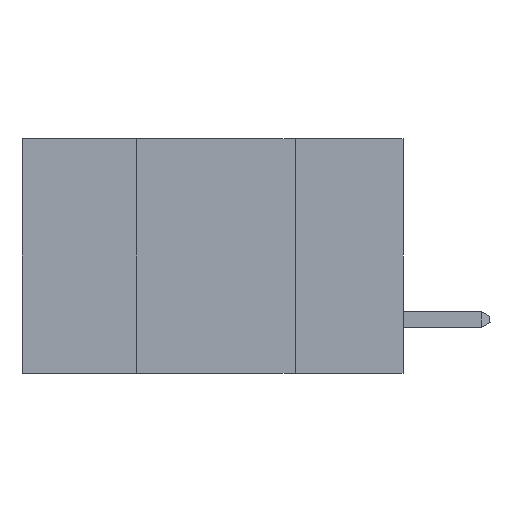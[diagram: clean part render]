
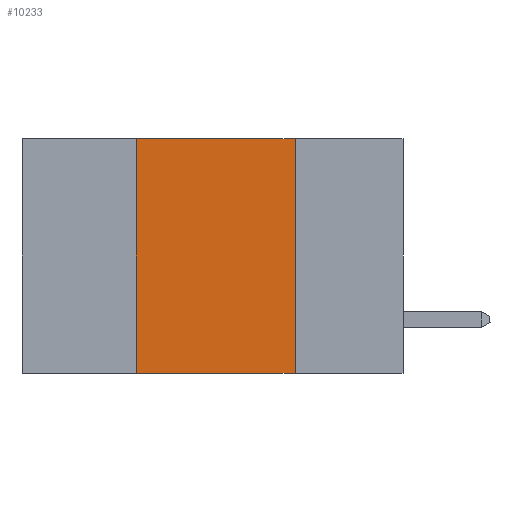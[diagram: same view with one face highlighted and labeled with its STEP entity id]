
A CAD part, left-side view. The second image highlights one B-rep face of the part: STEP entity #10233.
In plain terms, the highlighted planar face has unit normal (-1, 0, 0).
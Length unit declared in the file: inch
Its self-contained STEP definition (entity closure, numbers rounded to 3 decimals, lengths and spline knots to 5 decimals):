
#122 = CARTESIAN_POINT ( 'NONE',  ( 0., 0.42, 0. ) ) ;
#280 = LINE ( 'NONE', #984, #10540 ) ;
#643 = DIRECTION ( 'NONE',  ( 1., 0., 0. ) ) ;
#984 = CARTESIAN_POINT ( 'NONE',  ( 0., 0.6, -0.37 ) ) ;
#1367 = VECTOR ( 'NONE', #7132, 39.37008 ) ;
#1534 = CARTESIAN_POINT ( 'NONE',  ( 0., 0.6, 0. ) ) ;
#1822 = ORIENTED_EDGE ( 'NONE', *, *, #8252, .F. ) ;
#2962 = VERTEX_POINT ( 'NONE', #122 ) ;
#3509 = CARTESIAN_POINT ( 'NONE',  ( 0., 0.17, 0. ) ) ;
#4547 = EDGE_CURVE ( 'NONE', #14179, #15267, #17227, .T. ) ;
#5082 = LINE ( 'NONE', #1534, #1367 ) ;
#5216 = LINE ( 'NONE', #10218, #15890 ) ;
#5718 = EDGE_CURVE ( 'NONE', #6297, #2962, #5216, .T. ) ;
#6101 = VECTOR ( 'NONE', #17978, 39.37008 ) ;
#6152 = PLANE ( 'NONE',  #7188 ) ;
#6297 = VERTEX_POINT ( 'NONE', #12983 ) ;
#7132 = DIRECTION ( 'NONE',  ( 0., -1., 0. ) ) ;
#7188 = AXIS2_PLACEMENT_3D ( 'NONE', #17367, #643, #10384 ) ;
#8252 = EDGE_CURVE ( 'NONE', #2962, #14179, #5082, .T. ) ;
#8772 = EDGE_LOOP ( 'NONE', ( #8793, #1822, #12956, #16664 ) ) ;
#8793 = ORIENTED_EDGE ( 'NONE', *, *, #4547, .F. ) ;
#10218 = CARTESIAN_POINT ( 'NONE',  ( 0., 0.42, 0. ) ) ;
#10233 = ADVANCED_FACE ( 'NONE', ( #11733 ), #6152, .F. ) ;
#10384 = DIRECTION ( 'NONE',  ( 0., 0., -1. ) ) ;
#10540 = VECTOR ( 'NONE', #13561, 39.37008 ) ;
#11564 = DIRECTION ( 'NONE',  ( 0., 0., 1. ) ) ;
#11733 = FACE_OUTER_BOUND ( 'NONE', #8772, .T. ) ;
#12605 = EDGE_CURVE ( 'NONE', #6297, #15267, #280, .T. ) ;
#12956 = ORIENTED_EDGE ( 'NONE', *, *, #5718, .F. ) ;
#12983 = CARTESIAN_POINT ( 'NONE',  ( 0., 0.42, -0.37 ) ) ;
#13561 = DIRECTION ( 'NONE',  ( 0., -1., 0. ) ) ;
#14179 = VERTEX_POINT ( 'NONE', #3509 ) ;
#15267 = VERTEX_POINT ( 'NONE', #17270 ) ;
#15890 = VECTOR ( 'NONE', #11564, 39.37008 ) ;
#16599 = CARTESIAN_POINT ( 'NONE',  ( 0., 0.17, 0. ) ) ;
#16664 = ORIENTED_EDGE ( 'NONE', *, *, #12605, .T. ) ;
#17227 = LINE ( 'NONE', #16599, #6101 ) ;
#17270 = CARTESIAN_POINT ( 'NONE',  ( 0., 0.17, -0.37 ) ) ;
#17367 = CARTESIAN_POINT ( 'NONE',  ( 0., 0.6, 0. ) ) ;
#17978 = DIRECTION ( 'NONE',  ( 0., 0., -1. ) ) ;
